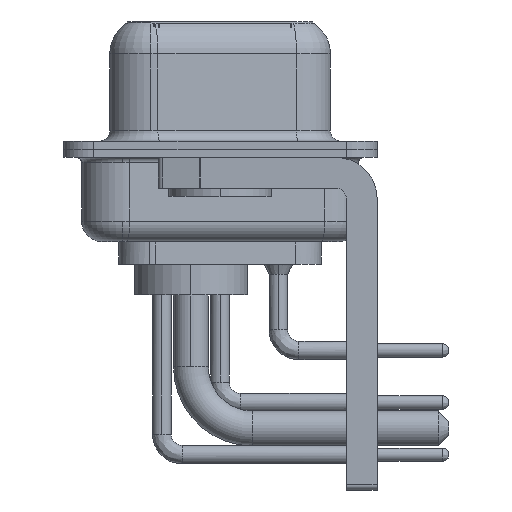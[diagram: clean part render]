
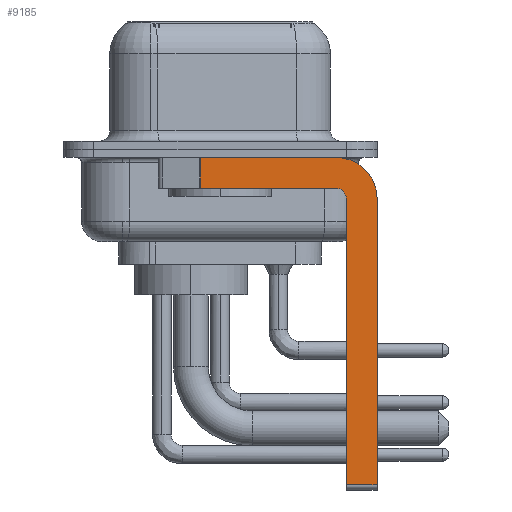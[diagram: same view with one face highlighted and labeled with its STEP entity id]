
A CAD part, left-side view. The second image highlights one B-rep face of the part: STEP entity #9185.
In plain terms, the highlighted planar face has unit normal (-1, 0, 0).
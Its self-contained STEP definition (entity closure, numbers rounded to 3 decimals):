
#602 = VERTEX_POINT ( 'NONE', #15562 ) ;
#921 = CARTESIAN_POINT ( 'NONE',  ( -2.9, 0.978, -0.4 ) ) ;
#1433 = CARTESIAN_POINT ( 'NONE',  ( -2.9, 0.978, -1.9 ) ) ;
#1489 = EDGE_CURVE ( 'NONE', #17054, #602, #7358, .T. ) ;
#2258 = CARTESIAN_POINT ( 'NONE',  ( -2.9, -5.65, -1.9 ) ) ;
#3467 = VECTOR ( 'NONE', #32760, 1000. ) ;
#3849 = DIRECTION ( 'NONE',  ( 0., 0., -1. ) ) ;
#3939 = VECTOR ( 'NONE', #28299, 1000. ) ;
#4190 = DIRECTION ( 'NONE',  ( -1., 0., 0. ) ) ;
#4916 = VERTEX_POINT ( 'NONE', #2258 ) ;
#5384 = DIRECTION ( 'NONE',  ( 1., 0., 0. ) ) ;
#5719 = CARTESIAN_POINT ( 'NONE',  ( -2.9, -5.65, -16.35 ) ) ;
#5931 = EDGE_CURVE ( 'NONE', #17054, #15488, #6498, .T. ) ;
#6498 = LINE ( 'NONE', #1433, #3467 ) ;
#6518 = CARTESIAN_POINT ( 'NONE',  ( -2.9, 0.978, -1.9 ) ) ;
#6758 = ORIENTED_EDGE ( 'NONE', *, *, #18224, .T. ) ;
#6857 = ORIENTED_EDGE ( 'NONE', *, *, #18036, .F. ) ;
#7137 = LINE ( 'NONE', #25651, #19500 ) ;
#7358 = LINE ( 'NONE', #12585, #23982 ) ;
#7755 = CARTESIAN_POINT ( 'NONE',  ( -2.9, -7.65, -16.35 ) ) ;
#8484 = VECTOR ( 'NONE', #3849, 1000. ) ;
#9036 = CARTESIAN_POINT ( 'NONE',  ( -2.9, -6.15, -2.4 ) ) ;
#9185 = ADVANCED_FACE ( 'NONE', ( #28231 ), #26876, .F. ) ;
#10381 = CARTESIAN_POINT ( 'NONE',  ( -2.9, -7.65, -2.4 ) ) ;
#11641 = LINE ( 'NONE', #21914, #17360 ) ;
#12585 = CARTESIAN_POINT ( 'NONE',  ( -2.9, 3., -0.4 ) ) ;
#12692 = DIRECTION ( 'NONE',  ( 0., 1., 0. ) ) ;
#13265 = CARTESIAN_POINT ( 'NONE',  ( -2.9, -6.15, -16.35 ) ) ;
#13462 = CARTESIAN_POINT ( 'NONE',  ( -2.9, -5.65, -2.4 ) ) ;
#13977 = VERTEX_POINT ( 'NONE', #13265 ) ;
#14458 = CARTESIAN_POINT ( 'NONE',  ( -2.9, -5.65, -2.4 ) ) ;
#14778 = DIRECTION ( 'NONE',  ( 0., -1., 0. ) ) ;
#14878 = AXIS2_PLACEMENT_3D ( 'NONE', #13462, #5384, #15644 ) ;
#15317 = CIRCLE ( 'NONE', #17491, 0.5 ) ;
#15417 = CIRCLE ( 'NONE', #14878, 2. ) ;
#15488 = VERTEX_POINT ( 'NONE', #6518 ) ;
#15562 = CARTESIAN_POINT ( 'NONE',  ( -2.9, -5.65, -0.4 ) ) ;
#15590 = ORIENTED_EDGE ( 'NONE', *, *, #1489, .F. ) ;
#15644 = DIRECTION ( 'NONE',  ( 0., 0., -1. ) ) ;
#15850 = EDGE_LOOP ( 'NONE', ( #15590, #26051, #23662, #32012, #6857, #6758, #16143, #26715 ) ) ;
#16119 = EDGE_CURVE ( 'NONE', #4916, #15488, #7137, .T. ) ;
#16143 = ORIENTED_EDGE ( 'NONE', *, *, #22649, .F. ) ;
#16717 = VERTEX_POINT ( 'NONE', #7755 ) ;
#17054 = VERTEX_POINT ( 'NONE', #921 ) ;
#17360 = VECTOR ( 'NONE', #24596, 1000. ) ;
#17491 = AXIS2_PLACEMENT_3D ( 'NONE', #14458, #4190, #29613 ) ;
#18036 = EDGE_CURVE ( 'NONE', #13977, #24426, #11641, .T. ) ;
#18224 = EDGE_CURVE ( 'NONE', #13977, #16717, #31300, .T. ) ;
#19147 = DIRECTION ( 'NONE',  ( 0., 0., -1. ) ) ;
#19500 = VECTOR ( 'NONE', #12692, 1000. ) ;
#19567 = VERTEX_POINT ( 'NONE', #10381 ) ;
#21867 = AXIS2_PLACEMENT_3D ( 'NONE', #31744, #24345, #19147 ) ;
#21914 = CARTESIAN_POINT ( 'NONE',  ( -2.9, -6.15, -16.6 ) ) ;
#22649 = EDGE_CURVE ( 'NONE', #19567, #16717, #26916, .T. ) ;
#23662 = ORIENTED_EDGE ( 'NONE', *, *, #16119, .F. ) ;
#23982 = VECTOR ( 'NONE', #14778, 1000. ) ;
#24345 = DIRECTION ( 'NONE',  ( 1., 0., 0. ) ) ;
#24426 = VERTEX_POINT ( 'NONE', #9036 ) ;
#24596 = DIRECTION ( 'NONE',  ( 0., 0., 1. ) ) ;
#25651 = CARTESIAN_POINT ( 'NONE',  ( -2.9, -5.65, -1.9 ) ) ;
#26051 = ORIENTED_EDGE ( 'NONE', *, *, #5931, .T. ) ;
#26715 = ORIENTED_EDGE ( 'NONE', *, *, #28519, .F. ) ;
#26876 = PLANE ( 'NONE',  #21867 ) ;
#26916 = LINE ( 'NONE', #29106, #8484 ) ;
#27448 = EDGE_CURVE ( 'NONE', #24426, #4916, #15317, .T. ) ;
#28231 = FACE_OUTER_BOUND ( 'NONE', #15850, .T. ) ;
#28299 = DIRECTION ( 'NONE',  ( 0., -1., 0. ) ) ;
#28519 = EDGE_CURVE ( 'NONE', #602, #19567, #15417, .T. ) ;
#29106 = CARTESIAN_POINT ( 'NONE',  ( -2.9, -7.65, -2.4 ) ) ;
#29613 = DIRECTION ( 'NONE',  ( 0., 0., 1. ) ) ;
#31300 = LINE ( 'NONE', #5719, #3939 ) ;
#31744 = CARTESIAN_POINT ( 'NONE',  ( -2.9, -5.65, -2.4 ) ) ;
#32012 = ORIENTED_EDGE ( 'NONE', *, *, #27448, .F. ) ;
#32760 = DIRECTION ( 'NONE',  ( 0., 0., -1. ) ) ;
